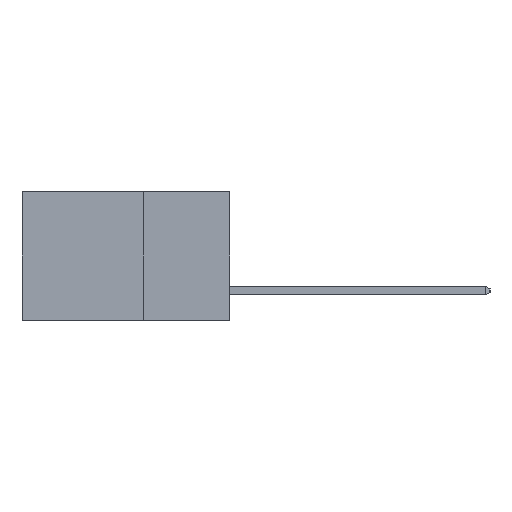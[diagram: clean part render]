
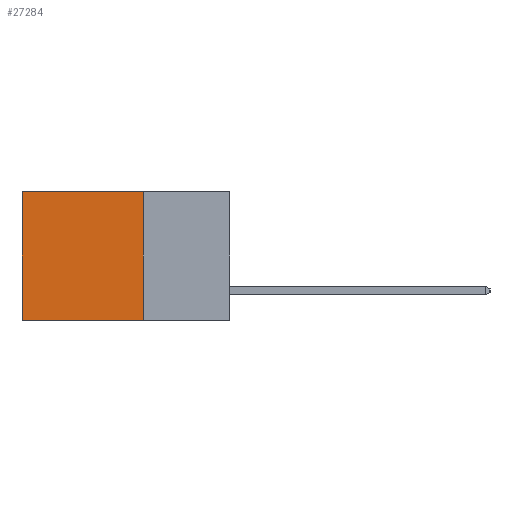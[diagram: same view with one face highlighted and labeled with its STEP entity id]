
A CAD part, left-side view. The second image highlights one B-rep face of the part: STEP entity #27284.
In plain terms, the highlighted planar face has unit normal (-1, 0, 0).
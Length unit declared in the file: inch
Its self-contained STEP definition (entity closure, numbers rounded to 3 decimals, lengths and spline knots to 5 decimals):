
#7 = ORIENTED_EDGE ( 'NONE', *, *, #1664, .F. ) ;
#496 = DIRECTION ( 'NONE',  ( 0., 0., -1. ) ) ;
#597 = CARTESIAN_POINT ( 'NONE',  ( 0.298, 0.25, -0.37 ) ) ;
#1664 = EDGE_CURVE ( 'NONE', #21181, #22413, #12872, .T. ) ;
#1842 = ORIENTED_EDGE ( 'NONE', *, *, #4951, .T. ) ;
#2219 = EDGE_LOOP ( 'NONE', ( #13283, #19312, #7, #1842 ) ) ;
#2789 = DIRECTION ( 'NONE',  ( 0., 1., 0. ) ) ;
#3027 = CARTESIAN_POINT ( 'NONE',  ( 0.298, 0.6, 0. ) ) ;
#3156 = VECTOR ( 'NONE', #13023, 39.37008 ) ;
#3231 = DIRECTION ( 'NONE',  ( 1., 0., 0. ) ) ;
#4633 = VECTOR ( 'NONE', #4755, 39.37008 ) ;
#4755 = DIRECTION ( 'NONE',  ( 0., 0., -1. ) ) ;
#4951 = EDGE_CURVE ( 'NONE', #21181, #25409, #9034, .T. ) ;
#5046 = CARTESIAN_POINT ( 'NONE',  ( 0.298, 0.25, -0.37 ) ) ;
#5059 = AXIS2_PLACEMENT_3D ( 'NONE', #16389, #3231, #18570 ) ;
#6985 = CARTESIAN_POINT ( 'NONE',  ( 0.298, 0.6, 0. ) ) ;
#7602 = VERTEX_POINT ( 'NONE', #13434 ) ;
#9034 = LINE ( 'NONE', #10859, #3156 ) ;
#9125 = LINE ( 'NONE', #5046, #19984 ) ;
#9627 = EDGE_CURVE ( 'NONE', #22413, #7602, #9125, .T. ) ;
#10187 = FACE_OUTER_BOUND ( 'NONE', #2219, .T. ) ;
#10859 = CARTESIAN_POINT ( 'NONE',  ( 0.298, 0.25, 0. ) ) ;
#12872 = LINE ( 'NONE', #26348, #17938 ) ;
#13023 = DIRECTION ( 'NONE',  ( 0., 1., 0. ) ) ;
#13283 = ORIENTED_EDGE ( 'NONE', *, *, #14037, .T. ) ;
#13434 = CARTESIAN_POINT ( 'NONE',  ( 0.298, 0.6, -0.37 ) ) ;
#14037 = EDGE_CURVE ( 'NONE', #25409, #7602, #16292, .T. ) ;
#16292 = LINE ( 'NONE', #6985, #4633 ) ;
#16389 = CARTESIAN_POINT ( 'NONE',  ( 0.298, 0.25, 0. ) ) ;
#17631 = CARTESIAN_POINT ( 'NONE',  ( 0.298, 0.25, 0. ) ) ;
#17938 = VECTOR ( 'NONE', #496, 39.37008 ) ;
#18570 = DIRECTION ( 'NONE',  ( 0., 0., -1. ) ) ;
#19312 = ORIENTED_EDGE ( 'NONE', *, *, #9627, .F. ) ;
#19984 = VECTOR ( 'NONE', #2789, 39.37008 ) ;
#21181 = VERTEX_POINT ( 'NONE', #17631 ) ;
#22413 = VERTEX_POINT ( 'NONE', #597 ) ;
#25409 = VERTEX_POINT ( 'NONE', #3027 ) ;
#26348 = CARTESIAN_POINT ( 'NONE',  ( 0.298, 0.25, 0. ) ) ;
#26949 = PLANE ( 'NONE',  #5059 ) ;
#27284 = ADVANCED_FACE ( 'NONE', ( #10187 ), #26949, .F. ) ;
